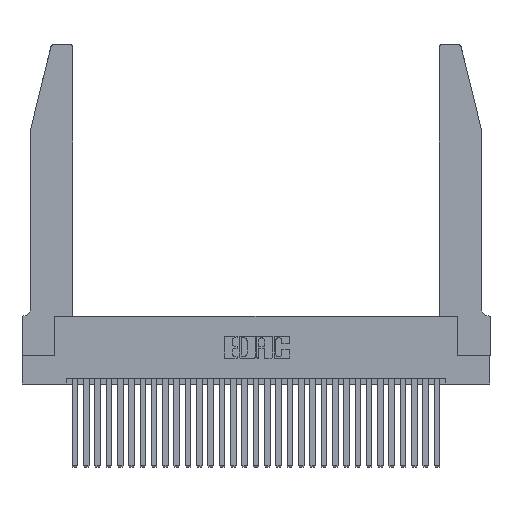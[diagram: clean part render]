
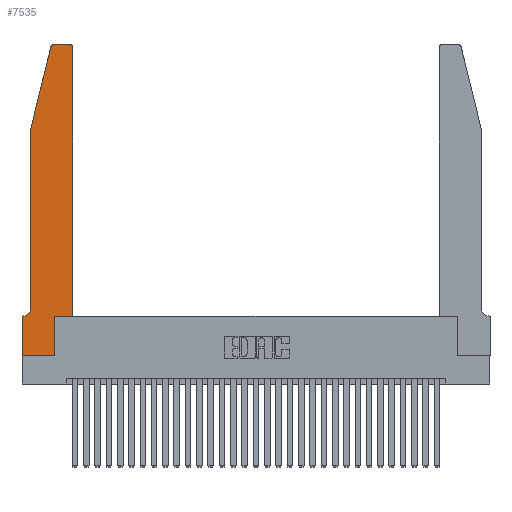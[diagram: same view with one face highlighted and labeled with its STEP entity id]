
A CAD part, top view. The second image highlights one B-rep face of the part: STEP entity #7535.
In plain terms, the highlighted planar face has unit normal (0, 0, 1).
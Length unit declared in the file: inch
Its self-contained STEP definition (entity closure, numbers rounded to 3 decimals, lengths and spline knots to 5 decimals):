
#148 = DIRECTION ( 'NONE',  ( 0., -1., 0. ) ) ;
#163 = CARTESIAN_POINT ( 'NONE',  ( 0.2605, 2.75, 0.37 ) ) ;
#474 = CARTESIAN_POINT ( 'NONE',  ( 0.25487, 2.72718, 0.37 ) ) ;
#699 = ORIENTED_EDGE ( 'NONE', *, *, #21275, .T. ) ;
#737 = AXIS2_PLACEMENT_3D ( 'NONE', #1028, #18335, #3553 ) ;
#862 = CARTESIAN_POINT ( 'NONE',  ( 0.4205, 2.75, 0.37 ) ) ;
#1028 = CARTESIAN_POINT ( 'NONE',  ( 0.284, 2.72, 0.37 ) ) ;
#1130 = DIRECTION ( 'NONE',  ( 1., 0., 0. ) ) ;
#1132 = LINE ( 'NONE', #22415, #20078 ) ;
#1244 = CARTESIAN_POINT ( 'NONE',  ( 0.284, 2.75, 0.37 ) ) ;
#1904 = LINE ( 'NONE', #14888, #27179 ) ;
#1999 = VECTOR ( 'NONE', #3113, 39.37008 ) ;
#2063 = AXIS2_PLACEMENT_3D ( 'NONE', #31568, #17142, #2329 ) ;
#2329 = DIRECTION ( 'NONE',  ( 1., 0., 0. ) ) ;
#2681 = CARTESIAN_POINT ( 'NONE',  ( 0.2865, 0., 0.37 ) ) ;
#2887 = LINE ( 'NONE', #22991, #7238 ) ;
#2906 = ORIENTED_EDGE ( 'NONE', *, *, #26860, .T. ) ;
#3113 = DIRECTION ( 'NONE',  ( 0., 1., 0. ) ) ;
#3553 = DIRECTION ( 'NONE',  ( 1., 0., 0. ) ) ;
#3717 = CARTESIAN_POINT ( 'NONE',  ( 0., 0.35, 0.37 ) ) ;
#3826 = VERTEX_POINT ( 'NONE', #7591 ) ;
#3953 = CARTESIAN_POINT ( 'NONE',  ( 0.4505, 0.35, 0.37 ) ) ;
#4107 = VERTEX_POINT ( 'NONE', #10973 ) ;
#5209 = EDGE_CURVE ( 'NONE', #14877, #3826, #19301, .T. ) ;
#5684 = CARTESIAN_POINT ( 'NONE',  ( 0.0755, 0.35, 0.37 ) ) ;
#5960 = ORIENTED_EDGE ( 'NONE', *, *, #28681, .T. ) ;
#5977 = VERTEX_POINT ( 'NONE', #9898 ) ;
#6514 = DIRECTION ( 'NONE',  ( 0., 1., 0. ) ) ;
#7152 = VECTOR ( 'NONE', #15015, 39.37008 ) ;
#7238 = VECTOR ( 'NONE', #25394, 39.37008 ) ;
#7395 = VERTEX_POINT ( 'NONE', #862 ) ;
#7535 = ADVANCED_FACE ( 'NONE', ( #11475 ), #23463, .T. ) ;
#7591 = CARTESIAN_POINT ( 'NONE',  ( 0.0755, 0.42, 0.37 ) ) ;
#7609 = CARTESIAN_POINT ( 'NONE',  ( 0.0055, 0.42, 0.37 ) ) ;
#7872 = LINE ( 'NONE', #17909, #1999 ) ;
#7935 = VERTEX_POINT ( 'NONE', #18025 ) ;
#8590 = CARTESIAN_POINT ( 'NONE',  ( 0., 0., 0.37 ) ) ;
#8683 = AXIS2_PLACEMENT_3D ( 'NONE', #7609, #24618, #10049 ) ;
#9898 = CARTESIAN_POINT ( 'NONE',  ( 0.2865, 0.35, 0.37 ) ) ;
#10049 = DIRECTION ( 'NONE',  ( -1., 0., 0. ) ) ;
#10257 = VECTOR ( 'NONE', #1130, 39.37008 ) ;
#10385 = CARTESIAN_POINT ( 'NONE',  ( 0., 0., 0.37 ) ) ;
#10553 = VERTEX_POINT ( 'NONE', #1244 ) ;
#10973 = CARTESIAN_POINT ( 'NONE',  ( 0.4505, 2.72, 0.37 ) ) ;
#11291 = DIRECTION ( 'NONE',  ( 0., 0., 1. ) ) ;
#11381 = ORIENTED_EDGE ( 'NONE', *, *, #23856, .T. ) ;
#11475 = FACE_OUTER_BOUND ( 'NONE', #12006, .T. ) ;
#12006 = EDGE_LOOP ( 'NONE', ( #699, #14726, #2906, #16046, #24431, #29514, #21890, #23013, #5960, #11381, #20967, #17550 ) ) ;
#13038 = DIRECTION ( 'NONE',  ( 0., -1., 0. ) ) ;
#13089 = LINE ( 'NONE', #5684, #18096 ) ;
#13298 = VERTEX_POINT ( 'NONE', #2681 ) ;
#13499 = VECTOR ( 'NONE', #13038, 39.37008 ) ;
#13641 = LINE ( 'NONE', #163, #7152 ) ;
#14073 = VECTOR ( 'NONE', #6514, 39.37008 ) ;
#14427 = VERTEX_POINT ( 'NONE', #21352 ) ;
#14726 = ORIENTED_EDGE ( 'NONE', *, *, #14892, .T. ) ;
#14762 = VERTEX_POINT ( 'NONE', #474 ) ;
#14877 = VERTEX_POINT ( 'NONE', #18116 ) ;
#14888 = CARTESIAN_POINT ( 'NONE',  ( 0., 0., 0.37 ) ) ;
#14892 = EDGE_CURVE ( 'NONE', #10553, #14762, #15514, .T. ) ;
#15015 = DIRECTION ( 'NONE',  ( -1., 0., 0. ) ) ;
#15514 = CIRCLE ( 'NONE', #737, 0.03 ) ;
#15518 = CARTESIAN_POINT ( 'NONE',  ( 0.0755, 2., 0.37 ) ) ;
#15536 = AXIS2_PLACEMENT_3D ( 'NONE', #3717, #11291, #28291 ) ;
#16046 = ORIENTED_EDGE ( 'NONE', *, *, #5209, .T. ) ;
#16611 = EDGE_CURVE ( 'NONE', #7935, #23166, #1904, .T. ) ;
#17038 = EDGE_CURVE ( 'NONE', #4107, #7395, #21554, .T. ) ;
#17142 = DIRECTION ( 'NONE',  ( 0., 0., 1. ) ) ;
#17550 = ORIENTED_EDGE ( 'NONE', *, *, #17038, .T. ) ;
#17909 = CARTESIAN_POINT ( 'NONE',  ( 0.2865, 0.35, 0.37 ) ) ;
#18025 = CARTESIAN_POINT ( 'NONE',  ( 0., 0.35, 0.37 ) ) ;
#18096 = VECTOR ( 'NONE', #22804, 39.37008 ) ;
#18116 = CARTESIAN_POINT ( 'NONE',  ( 0.0755, 2., 0.37 ) ) ;
#18335 = DIRECTION ( 'NONE',  ( 0., 0., 1. ) ) ;
#19194 = VERTEX_POINT ( 'NONE', #29926 ) ;
#19301 = LINE ( 'NONE', #15518, #13499 ) ;
#20078 = VECTOR ( 'NONE', #24814, 39.37008 ) ;
#20245 = EDGE_CURVE ( 'NONE', #23166, #13298, #23259, .T. ) ;
#20594 = LINE ( 'NONE', #3953, #14073 ) ;
#20967 = ORIENTED_EDGE ( 'NONE', *, *, #27505, .T. ) ;
#21275 = EDGE_CURVE ( 'NONE', #7395, #10553, #13641, .T. ) ;
#21352 = CARTESIAN_POINT ( 'NONE',  ( 0.0055, 0.35, 0.37 ) ) ;
#21554 = CIRCLE ( 'NONE', #2063, 0.03 ) ;
#21890 = ORIENTED_EDGE ( 'NONE', *, *, #16611, .T. ) ;
#22415 = CARTESIAN_POINT ( 'NONE',  ( 0.4505, 0.35, 0.37 ) ) ;
#22804 = DIRECTION ( 'NONE',  ( -1., 0., 0. ) ) ;
#22991 = CARTESIAN_POINT ( 'NONE',  ( 0.0755, 2., 0.37 ) ) ;
#23013 = ORIENTED_EDGE ( 'NONE', *, *, #20245, .T. ) ;
#23166 = VERTEX_POINT ( 'NONE', #10385 ) ;
#23259 = LINE ( 'NONE', #8590, #10257 ) ;
#23463 = PLANE ( 'NONE',  #15536 ) ;
#23856 = EDGE_CURVE ( 'NONE', #5977, #19194, #1132, .T. ) ;
#24431 = ORIENTED_EDGE ( 'NONE', *, *, #25672, .T. ) ;
#24594 = EDGE_CURVE ( 'NONE', #14427, #7935, #13089, .T. ) ;
#24618 = DIRECTION ( 'NONE',  ( 0., 0., -1. ) ) ;
#24814 = DIRECTION ( 'NONE',  ( 1., 0., 0. ) ) ;
#25394 = DIRECTION ( 'NONE',  ( -0.239, -0.971, 0. ) ) ;
#25672 = EDGE_CURVE ( 'NONE', #3826, #14427, #27837, .T. ) ;
#26860 = EDGE_CURVE ( 'NONE', #14762, #14877, #2887, .T. ) ;
#27179 = VECTOR ( 'NONE', #148, 39.37008 ) ;
#27505 = EDGE_CURVE ( 'NONE', #19194, #4107, #20594, .T. ) ;
#27837 = CIRCLE ( 'NONE', #8683, 0.07 ) ;
#28291 = DIRECTION ( 'NONE',  ( 1., 0., 0. ) ) ;
#28681 = EDGE_CURVE ( 'NONE', #13298, #5977, #7872, .T. ) ;
#29514 = ORIENTED_EDGE ( 'NONE', *, *, #24594, .T. ) ;
#29926 = CARTESIAN_POINT ( 'NONE',  ( 0.4505, 0.35, 0.37 ) ) ;
#31568 = CARTESIAN_POINT ( 'NONE',  ( 0.4205, 2.72, 0.37 ) ) ;
